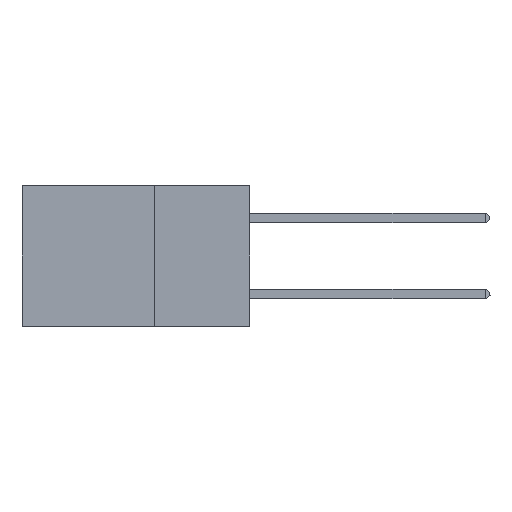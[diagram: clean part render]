
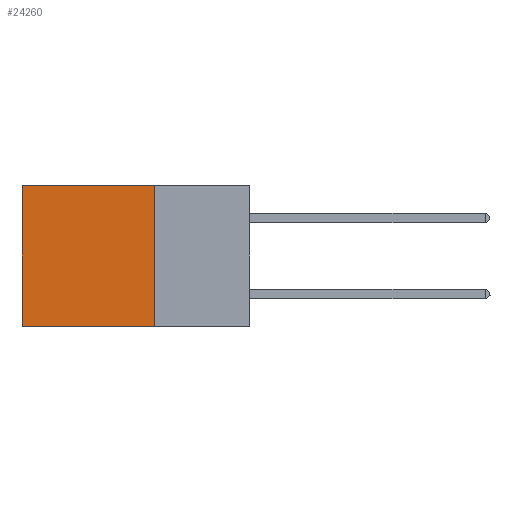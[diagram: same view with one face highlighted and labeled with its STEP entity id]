
A CAD part, left-side view. The second image highlights one B-rep face of the part: STEP entity #24260.
In plain terms, the highlighted planar face has unit normal (-1, 0, 0).
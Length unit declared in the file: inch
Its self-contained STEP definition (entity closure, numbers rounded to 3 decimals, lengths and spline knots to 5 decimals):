
#1421 = VECTOR ( 'NONE', #23110, 39.37008 ) ;
#2646 = CARTESIAN_POINT ( 'NONE',  ( 0.2875, 0.25, -0.37 ) ) ;
#2755 = EDGE_CURVE ( 'NONE', #35902, #28123, #18372, .T. ) ;
#4706 = CARTESIAN_POINT ( 'NONE',  ( 0.2875, 0.25, 0. ) ) ;
#5579 = CARTESIAN_POINT ( 'NONE',  ( 0.2875, 0.6, 0. ) ) ;
#6174 = VERTEX_POINT ( 'NONE', #42037 ) ;
#8066 = PLANE ( 'NONE',  #20082 ) ;
#11225 = CARTESIAN_POINT ( 'NONE',  ( 0.2875, 0.6, 0. ) ) ;
#11468 = LINE ( 'NONE', #5579, #45926 ) ;
#13827 = ORIENTED_EDGE ( 'NONE', *, *, #43763, .F. ) ;
#15334 = VECTOR ( 'NONE', #20983, 39.37008 ) ;
#16976 = CARTESIAN_POINT ( 'NONE',  ( 0.2875, 0.6, -0.37 ) ) ;
#17872 = CARTESIAN_POINT ( 'NONE',  ( 0.2875, 0.25, 0. ) ) ;
#18068 = EDGE_LOOP ( 'NONE', ( #34920, #13827, #29374, #19414 ) ) ;
#18372 = LINE ( 'NONE', #4706, #43955 ) ;
#18474 = DIRECTION ( 'NONE',  ( 0., 0., -1. ) ) ;
#18964 = VERTEX_POINT ( 'NONE', #16976 ) ;
#19414 = ORIENTED_EDGE ( 'NONE', *, *, #2755, .T. ) ;
#20082 = AXIS2_PLACEMENT_3D ( 'NONE', #25618, #25779, #18474 ) ;
#20983 = DIRECTION ( 'NONE',  ( 0., 1., 0. ) ) ;
#21963 = LINE ( 'NONE', #41222, #1421 ) ;
#23110 = DIRECTION ( 'NONE',  ( 0., 0., -1. ) ) ;
#24137 = FACE_OUTER_BOUND ( 'NONE', #18068, .T. ) ;
#24260 = ADVANCED_FACE ( 'NONE', ( #24137 ), #8066, .F. ) ;
#24801 = LINE ( 'NONE', #2646, #15334 ) ;
#25618 = CARTESIAN_POINT ( 'NONE',  ( 0.2875, 0.25, 0. ) ) ;
#25779 = DIRECTION ( 'NONE',  ( 1., 0., 0. ) ) ;
#28123 = VERTEX_POINT ( 'NONE', #11225 ) ;
#29374 = ORIENTED_EDGE ( 'NONE', *, *, #38085, .F. ) ;
#30751 = DIRECTION ( 'NONE',  ( 0., 0., -1. ) ) ;
#34920 = ORIENTED_EDGE ( 'NONE', *, *, #43628, .T. ) ;
#35902 = VERTEX_POINT ( 'NONE', #17872 ) ;
#38085 = EDGE_CURVE ( 'NONE', #35902, #6174, #21963, .T. ) ;
#40551 = DIRECTION ( 'NONE',  ( 0., 1., 0. ) ) ;
#41222 = CARTESIAN_POINT ( 'NONE',  ( 0.2875, 0.25, 0. ) ) ;
#42037 = CARTESIAN_POINT ( 'NONE',  ( 0.2875, 0.25, -0.37 ) ) ;
#43628 = EDGE_CURVE ( 'NONE', #28123, #18964, #11468, .T. ) ;
#43763 = EDGE_CURVE ( 'NONE', #6174, #18964, #24801, .T. ) ;
#43955 = VECTOR ( 'NONE', #40551, 39.37008 ) ;
#45926 = VECTOR ( 'NONE', #30751, 39.37008 ) ;
